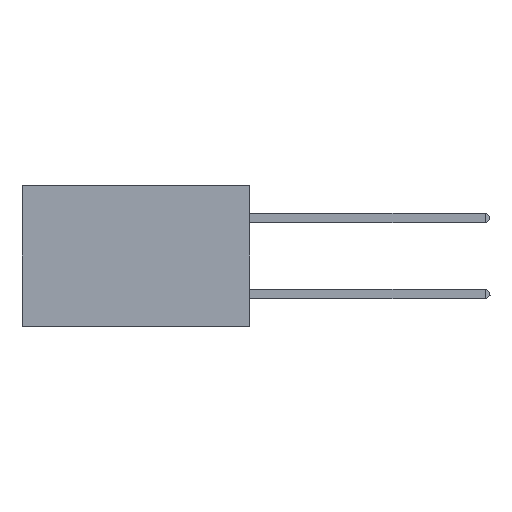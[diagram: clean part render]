
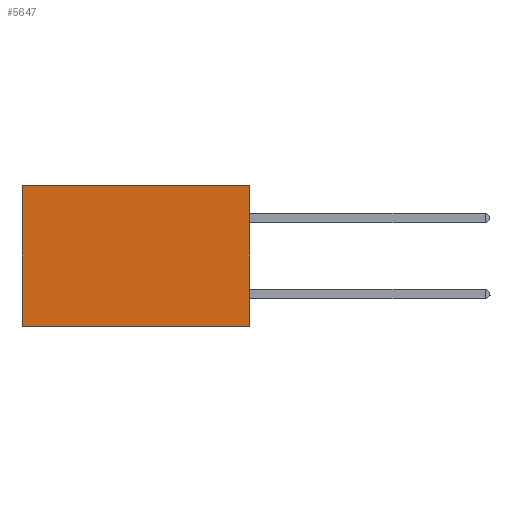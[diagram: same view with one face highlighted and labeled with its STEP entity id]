
A CAD part, left-side view. The second image highlights one B-rep face of the part: STEP entity #5647.
In plain terms, the highlighted planar face has unit normal (-1, 0, 0).
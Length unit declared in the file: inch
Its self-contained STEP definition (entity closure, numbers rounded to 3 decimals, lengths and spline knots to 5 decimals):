
#32 = FACE_OUTER_BOUND ( 'NONE', #23250, .T. ) ;
#246 = VECTOR ( 'NONE', #29379, 39.37008 ) ;
#262 = EDGE_CURVE ( 'NONE', #26618, #11727, #13188, .T. ) ;
#504 = EDGE_CURVE ( 'NONE', #4863, #11727, #13527, .T. ) ;
#1293 = ORIENTED_EDGE ( 'NONE', *, *, #26216, .T. ) ;
#1980 = CARTESIAN_POINT ( 'NONE',  ( 0.2875, 0., 0. ) ) ;
#2615 = CARTESIAN_POINT ( 'NONE',  ( 0.2875, 0.6, 0. ) ) ;
#4863 = VERTEX_POINT ( 'NONE', #26833 ) ;
#5647 = ADVANCED_FACE ( 'NONE', ( #32 ), #24413, .F. ) ;
#6370 = LINE ( 'NONE', #6389, #246 ) ;
#6389 = CARTESIAN_POINT ( 'NONE',  ( 0.2875, 0., 0. ) ) ;
#6815 = AXIS2_PLACEMENT_3D ( 'NONE', #8395, #17951, #8707 ) ;
#8149 = ORIENTED_EDGE ( 'NONE', *, *, #262, .T. ) ;
#8395 = CARTESIAN_POINT ( 'NONE',  ( 0.2875, 0., 0. ) ) ;
#8707 = DIRECTION ( 'NONE',  ( 0., 0., -1. ) ) ;
#11727 = VERTEX_POINT ( 'NONE', #24076 ) ;
#13188 = LINE ( 'NONE', #20491, #18497 ) ;
#13527 = LINE ( 'NONE', #20398, #28096 ) ;
#15245 = ORIENTED_EDGE ( 'NONE', *, *, #20265, .F. ) ;
#16583 = DIRECTION ( 'NONE',  ( 0., 0., -1. ) ) ;
#16690 = CARTESIAN_POINT ( 'NONE',  ( 0.2875, 0., 0. ) ) ;
#17169 = VERTEX_POINT ( 'NONE', #1980 ) ;
#17951 = DIRECTION ( 'NONE',  ( 1., 0., 0. ) ) ;
#18497 = VECTOR ( 'NONE', #20310, 39.37008 ) ;
#20265 = EDGE_CURVE ( 'NONE', #17169, #4863, #24269, .T. ) ;
#20310 = DIRECTION ( 'NONE',  ( 0., 0., -1. ) ) ;
#20398 = CARTESIAN_POINT ( 'NONE',  ( 0.2875, 0., -0.37 ) ) ;
#20491 = CARTESIAN_POINT ( 'NONE',  ( 0.2875, 0.6, 0. ) ) ;
#21017 = VECTOR ( 'NONE', #16583, 39.37008 ) ;
#21240 = DIRECTION ( 'NONE',  ( 0., 1., 0. ) ) ;
#23250 = EDGE_LOOP ( 'NONE', ( #8149, #25061, #15245, #1293 ) ) ;
#24076 = CARTESIAN_POINT ( 'NONE',  ( 0.2875, 0.6, -0.37 ) ) ;
#24269 = LINE ( 'NONE', #16690, #21017 ) ;
#24413 = PLANE ( 'NONE',  #6815 ) ;
#25061 = ORIENTED_EDGE ( 'NONE', *, *, #504, .F. ) ;
#26216 = EDGE_CURVE ( 'NONE', #17169, #26618, #6370, .T. ) ;
#26618 = VERTEX_POINT ( 'NONE', #2615 ) ;
#26833 = CARTESIAN_POINT ( 'NONE',  ( 0.2875, 0., -0.37 ) ) ;
#28096 = VECTOR ( 'NONE', #21240, 39.37008 ) ;
#29379 = DIRECTION ( 'NONE',  ( 0., 1., 0. ) ) ;
